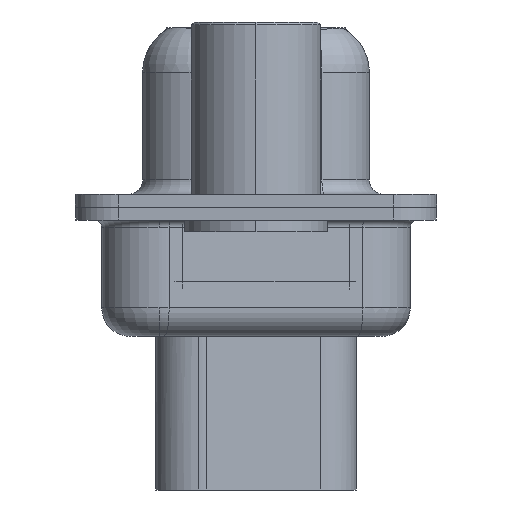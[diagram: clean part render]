
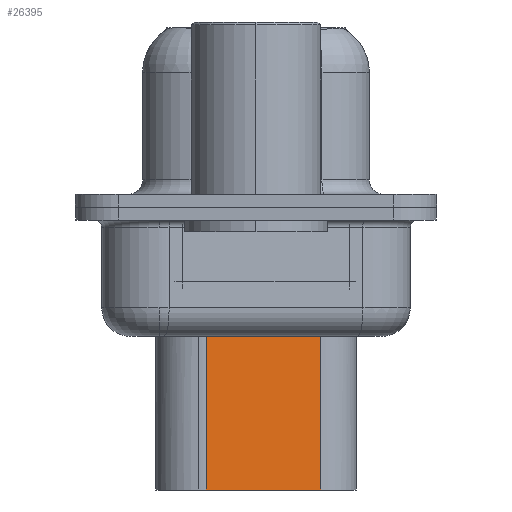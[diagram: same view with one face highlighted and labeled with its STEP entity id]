
A CAD part, left-side view. The second image highlights one B-rep face of the part: STEP entity #26395.
In plain terms, the highlighted planar face has unit normal (-0.985, -0.174, 0).
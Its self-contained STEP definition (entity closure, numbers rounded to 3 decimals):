
#569 = CARTESIAN_POINT ( 'NONE',  ( 4.524, 1.74, -3.975 ) ) ;
#2300 = DIRECTION ( 'NONE',  ( -0.985, -0.174, 0. ) ) ;
#4059 = EDGE_CURVE ( 'NONE', #18810, #32126, #30931, .T. ) ;
#5276 = EDGE_CURVE ( 'NONE', #30822, #32126, #11649, .T. ) ;
#5475 = LINE ( 'NONE', #7470, #14766 ) ;
#5511 = ORIENTED_EDGE ( 'NONE', *, *, #4059, .F. ) ;
#6036 = VECTOR ( 'NONE', #19091, 1000. ) ;
#7084 = DIRECTION ( 'NONE',  ( 0.174, -0.985, 0. ) ) ;
#7470 = CARTESIAN_POINT ( 'NONE',  ( 5.229, -2.26, -3.1 ) ) ;
#7903 = VERTEX_POINT ( 'NONE', #8758 ) ;
#8758 = CARTESIAN_POINT ( 'NONE',  ( 5.229, -2.26, -3.975 ) ) ;
#9148 = EDGE_CURVE ( 'NONE', #7903, #30822, #24152, .T. ) ;
#9964 = ORIENTED_EDGE ( 'NONE', *, *, #9148, .T. ) ;
#10813 = DIRECTION ( 'NONE',  ( -0.174, 0.985, 0. ) ) ;
#11228 = CARTESIAN_POINT ( 'NONE',  ( 4.524, 1.74, -9.85 ) ) ;
#11649 = LINE ( 'NONE', #18762, #6036 ) ;
#13277 = EDGE_CURVE ( 'NONE', #7903, #18810, #5475, .T. ) ;
#13922 = CARTESIAN_POINT ( 'NONE',  ( 5.229, -2.26, -9.85 ) ) ;
#14766 = VECTOR ( 'NONE', #14942, 1000. ) ;
#14893 = PLANE ( 'NONE',  #18582 ) ;
#14942 = DIRECTION ( 'NONE',  ( 0., 0., -1. ) ) ;
#15472 = CARTESIAN_POINT ( 'NONE',  ( 4.353, 2.709, -3.975 ) ) ;
#18582 = AXIS2_PLACEMENT_3D ( 'NONE', #30066, #2300, #7084 ) ;
#18762 = CARTESIAN_POINT ( 'NONE',  ( 4.524, 1.74, -3.1 ) ) ;
#18810 = VERTEX_POINT ( 'NONE', #13922 ) ;
#19091 = DIRECTION ( 'NONE',  ( 0., 0., -1. ) ) ;
#20634 = ORIENTED_EDGE ( 'NONE', *, *, #13277, .F. ) ;
#21203 = DIRECTION ( 'NONE',  ( -0.174, 0.985, 0. ) ) ;
#24152 = LINE ( 'NONE', #15472, #24606 ) ;
#24374 = VECTOR ( 'NONE', #10813, 1000. ) ;
#24606 = VECTOR ( 'NONE', #21203, 1000. ) ;
#24852 = EDGE_LOOP ( 'NONE', ( #20634, #9964, #32071, #5511 ) ) ;
#25842 = CARTESIAN_POINT ( 'NONE',  ( 4.524, 1.74, -9.85 ) ) ;
#26395 = ADVANCED_FACE ( 'NONE', ( #27262 ), #14893, .T. ) ;
#27262 = FACE_OUTER_BOUND ( 'NONE', #24852, .T. ) ;
#30066 = CARTESIAN_POINT ( 'NONE',  ( 4.524, 1.74, -3.1 ) ) ;
#30822 = VERTEX_POINT ( 'NONE', #569 ) ;
#30931 = LINE ( 'NONE', #25842, #24374 ) ;
#32071 = ORIENTED_EDGE ( 'NONE', *, *, #5276, .T. ) ;
#32126 = VERTEX_POINT ( 'NONE', #11228 ) ;
